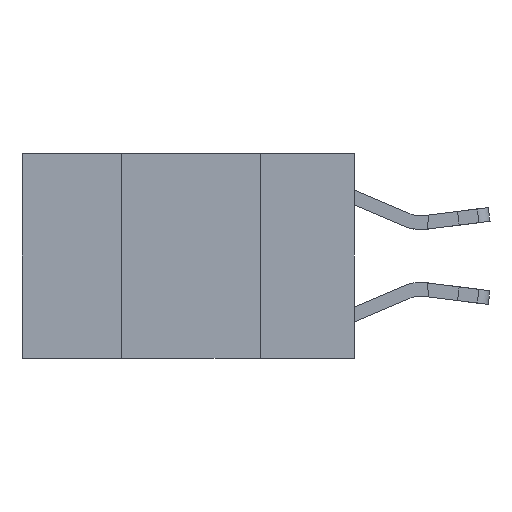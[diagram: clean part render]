
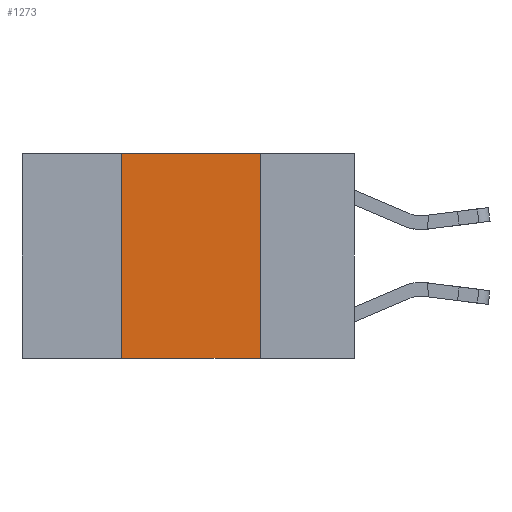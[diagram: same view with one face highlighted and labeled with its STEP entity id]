
A CAD part, left-side view. The second image highlights one B-rep face of the part: STEP entity #1273.
In plain terms, the highlighted planar face has unit normal (-1, 0, 0).
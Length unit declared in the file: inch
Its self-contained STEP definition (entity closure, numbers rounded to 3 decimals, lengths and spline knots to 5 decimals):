
#1273 = ADVANCED_FACE ( 'NONE', ( #15118 ), #5342, .F. ) ;
#1330 = DIRECTION ( 'NONE',  ( 0., 0., 1. ) ) ;
#3702 = VECTOR ( 'NONE', #14559, 39.37008 ) ;
#4624 = EDGE_CURVE ( 'NONE', #7425, #21858, #17299, .T. ) ;
#5342 = PLANE ( 'NONE',  #10890 ) ;
#5614 = EDGE_CURVE ( 'NONE', #22266, #12296, #21556, .T. ) ;
#6845 = VECTOR ( 'NONE', #13061, 39.37008 ) ;
#7085 = CARTESIAN_POINT ( 'NONE',  ( 0., 0.17, 0. ) ) ;
#7211 = DIRECTION ( 'NONE',  ( 1., 0., 0. ) ) ;
#7303 = ORIENTED_EDGE ( 'NONE', *, *, #5614, .T. ) ;
#7425 = VERTEX_POINT ( 'NONE', #10471 ) ;
#8911 = DIRECTION ( 'NONE',  ( 0., 0., -1. ) ) ;
#10471 = CARTESIAN_POINT ( 'NONE',  ( 0., 0.42, 0. ) ) ;
#10890 = AXIS2_PLACEMENT_3D ( 'NONE', #12695, #7211, #20111 ) ;
#10904 = VECTOR ( 'NONE', #8911, 39.37008 ) ;
#11619 = ORIENTED_EDGE ( 'NONE', *, *, #13979, .F. ) ;
#12296 = VERTEX_POINT ( 'NONE', #13450 ) ;
#12414 = CARTESIAN_POINT ( 'NONE',  ( 0., 0.42, 0. ) ) ;
#12695 = CARTESIAN_POINT ( 'NONE',  ( 0., 0.6, 0. ) ) ;
#13061 = DIRECTION ( 'NONE',  ( 0., -1., 0. ) ) ;
#13450 = CARTESIAN_POINT ( 'NONE',  ( 0., 0.17, -0.37 ) ) ;
#13979 = EDGE_CURVE ( 'NONE', #22266, #7425, #23004, .T. ) ;
#14053 = EDGE_CURVE ( 'NONE', #21858, #12296, #16997, .T. ) ;
#14559 = DIRECTION ( 'NONE',  ( 0., -1., 0. ) ) ;
#15118 = FACE_OUTER_BOUND ( 'NONE', #18150, .T. ) ;
#15981 = ORIENTED_EDGE ( 'NONE', *, *, #14053, .F. ) ;
#16424 = CARTESIAN_POINT ( 'NONE',  ( 0., 0.6, 0. ) ) ;
#16997 = LINE ( 'NONE', #7085, #10904 ) ;
#17299 = LINE ( 'NONE', #16424, #3702 ) ;
#17563 = VECTOR ( 'NONE', #1330, 39.37008 ) ;
#18150 = EDGE_LOOP ( 'NONE', ( #15981, #20852, #11619, #7303 ) ) ;
#18543 = CARTESIAN_POINT ( 'NONE',  ( 0., 0.6, -0.37 ) ) ;
#19639 = CARTESIAN_POINT ( 'NONE',  ( 0., 0.17, 0. ) ) ;
#20111 = DIRECTION ( 'NONE',  ( 0., 0., -1. ) ) ;
#20679 = CARTESIAN_POINT ( 'NONE',  ( 0., 0.42, -0.37 ) ) ;
#20852 = ORIENTED_EDGE ( 'NONE', *, *, #4624, .F. ) ;
#21556 = LINE ( 'NONE', #18543, #6845 ) ;
#21858 = VERTEX_POINT ( 'NONE', #19639 ) ;
#22266 = VERTEX_POINT ( 'NONE', #20679 ) ;
#23004 = LINE ( 'NONE', #12414, #17563 ) ;
